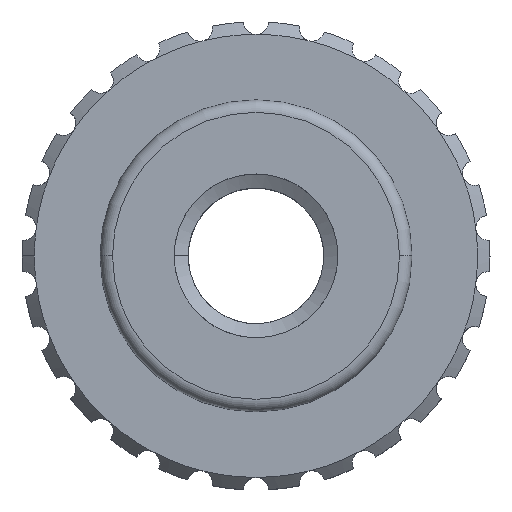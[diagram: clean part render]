
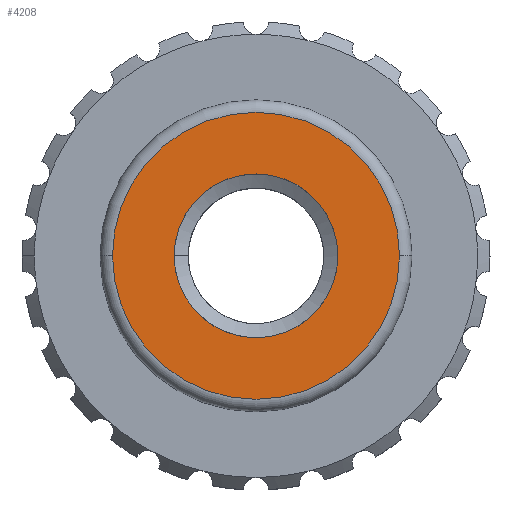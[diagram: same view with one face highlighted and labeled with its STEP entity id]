
A CAD part, top view. The second image highlights one B-rep face of the part: STEP entity #4208.
In plain terms, the highlighted planar face has unit normal (0, 0, 1).
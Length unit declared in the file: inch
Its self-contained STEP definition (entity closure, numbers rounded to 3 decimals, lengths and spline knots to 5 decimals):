
#192 = DIRECTION ( 'NONE',  ( 0., 0., 1. ) ) ;
#197 = EDGE_CURVE ( 'NONE', #5420, #1050, #3379, .T. ) ;
#239 = DIRECTION ( 'NONE',  ( 1., 0., 0. ) ) ;
#267 = EDGE_LOOP ( 'NONE', ( #635, #3992 ) ) ;
#350 = EDGE_CURVE ( 'NONE', #2161, #5169, #2797, .T. ) ;
#635 = ORIENTED_EDGE ( 'NONE', *, *, #4949, .T. ) ;
#649 = ORIENTED_EDGE ( 'NONE', *, *, #197, .F. ) ;
#754 = EDGE_CURVE ( 'NONE', #1050, #5420, #2732, .T. ) ;
#850 = AXIS2_PLACEMENT_3D ( 'NONE', #1979, #3273, #4635 ) ;
#1050 = VERTEX_POINT ( 'NONE', #4283 ) ;
#1136 = PLANE ( 'NONE',  #850 ) ;
#1481 = DIRECTION ( 'NONE',  ( 1., 0., 0. ) ) ;
#1552 = CARTESIAN_POINT ( 'NONE',  ( -0.84422, 1.00075, 0.25 ) ) ;
#1972 = AXIS2_PLACEMENT_3D ( 'NONE', #5022, #192, #1481 ) ;
#1979 = CARTESIAN_POINT ( 'NONE',  ( -0.84422, 1.00075, 0.25 ) ) ;
#2031 = CARTESIAN_POINT ( 'NONE',  ( -0.71297, 1.00075, 0.25 ) ) ;
#2161 = VERTEX_POINT ( 'NONE', #3398 ) ;
#2172 = ORIENTED_EDGE ( 'NONE', *, *, #754, .F. ) ;
#2398 = DIRECTION ( 'NONE',  ( 0., 0., 1. ) ) ;
#2470 = AXIS2_PLACEMENT_3D ( 'NONE', #1552, #2398, #239 ) ;
#2650 = AXIS2_PLACEMENT_3D ( 'NONE', #3912, #4349, #3530 ) ;
#2732 = CIRCLE ( 'NONE', #1972, 0.13125 ) ;
#2750 = AXIS2_PLACEMENT_3D ( 'NONE', #3394, #5616, #5543 ) ;
#2797 = CIRCLE ( 'NONE', #2650, 0.23 ) ;
#2883 = EDGE_LOOP ( 'NONE', ( #2172, #649 ) ) ;
#3273 = DIRECTION ( 'NONE',  ( 0., 0., 1. ) ) ;
#3379 = CIRCLE ( 'NONE', #2750, 0.13125 ) ;
#3394 = CARTESIAN_POINT ( 'NONE',  ( -0.84422, 1.00075, 0.25 ) ) ;
#3398 = CARTESIAN_POINT ( 'NONE',  ( -1.07422, 1.00075, 0.25 ) ) ;
#3530 = DIRECTION ( 'NONE',  ( 1., 0., 0. ) ) ;
#3831 = CIRCLE ( 'NONE', #2470, 0.23 ) ;
#3903 = FACE_BOUND ( 'NONE', #2883, .T. ) ;
#3912 = CARTESIAN_POINT ( 'NONE',  ( -0.84422, 1.00075, 0.25 ) ) ;
#3992 = ORIENTED_EDGE ( 'NONE', *, *, #350, .T. ) ;
#4208 = ADVANCED_FACE ( 'NONE', ( #4576, #3903 ), #1136, .T. ) ;
#4283 = CARTESIAN_POINT ( 'NONE',  ( -0.97547, 1.00075, 0.25 ) ) ;
#4349 = DIRECTION ( 'NONE',  ( 0., 0., 1. ) ) ;
#4576 = FACE_OUTER_BOUND ( 'NONE', #267, .T. ) ;
#4635 = DIRECTION ( 'NONE',  ( 1., 0., 0. ) ) ;
#4949 = EDGE_CURVE ( 'NONE', #5169, #2161, #3831, .T. ) ;
#5022 = CARTESIAN_POINT ( 'NONE',  ( -0.84422, 1.00075, 0.25 ) ) ;
#5169 = VERTEX_POINT ( 'NONE', #5222 ) ;
#5222 = CARTESIAN_POINT ( 'NONE',  ( -0.61422, 1.00075, 0.25 ) ) ;
#5420 = VERTEX_POINT ( 'NONE', #2031 ) ;
#5543 = DIRECTION ( 'NONE',  ( 1., 0., 0. ) ) ;
#5616 = DIRECTION ( 'NONE',  ( 0., 0., 1. ) ) ;
